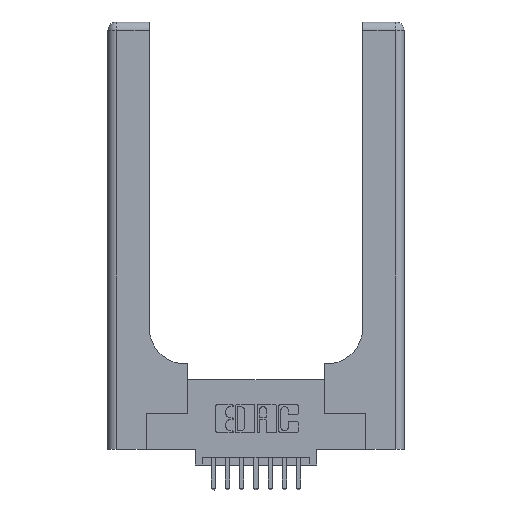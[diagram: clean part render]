
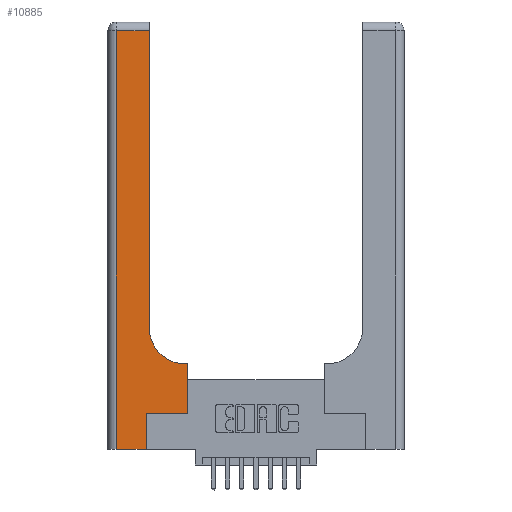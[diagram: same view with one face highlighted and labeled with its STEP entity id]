
A CAD part, top view. The second image highlights one B-rep face of the part: STEP entity #10885.
In plain terms, the highlighted planar face has unit normal (0, 0, 1).
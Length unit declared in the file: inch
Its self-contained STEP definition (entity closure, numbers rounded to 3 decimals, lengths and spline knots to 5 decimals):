
#163 = CARTESIAN_POINT ( 'NONE',  ( 0.2915, 0.85, 0.37 ) ) ;
#548 = VECTOR ( 'NONE', #11658, 39.37008 ) ;
#653 = EDGE_CURVE ( 'NONE', #9798, #8489, #15394, .T. ) ;
#676 = CARTESIAN_POINT ( 'NONE',  ( 0.5415, 0.6, 0.37 ) ) ;
#762 = DIRECTION ( 'NONE',  ( 0., 0., -1. ) ) ;
#998 = EDGE_CURVE ( 'NONE', #1137, #9798, #2732, .T. ) ;
#1020 = CARTESIAN_POINT ( 'NONE',  ( 0., 3., 0.37 ) ) ;
#1137 = VERTEX_POINT ( 'NONE', #5289 ) ;
#2451 = LINE ( 'NONE', #2873, #13931 ) ;
#2629 = CARTESIAN_POINT ( 'NONE',  ( 0., 0., 0.37 ) ) ;
#2639 = VECTOR ( 'NONE', #4273, 39.37008 ) ;
#2732 = LINE ( 'NONE', #12496, #13647 ) ;
#2873 = CARTESIAN_POINT ( 'NONE',  ( 0., 2.94, 0.37 ) ) ;
#3218 = CARTESIAN_POINT ( 'NONE',  ( 0.2915, 3., 0.37 ) ) ;
#3639 = CARTESIAN_POINT ( 'NONE',  ( 0.5585, 0.25, 0.37 ) ) ;
#3951 = CARTESIAN_POINT ( 'NONE',  ( 0.06, 0., 0.37 ) ) ;
#4054 = EDGE_CURVE ( 'NONE', #8489, #8367, #8633, .T. ) ;
#4134 = LINE ( 'NONE', #2629, #6196 ) ;
#4273 = DIRECTION ( 'NONE',  ( 0., -1., 0. ) ) ;
#4312 = CARTESIAN_POINT ( 'NONE',  ( 0.06, 3., 0.37 ) ) ;
#4530 = DIRECTION ( 'NONE',  ( 1., 0., 0. ) ) ;
#4960 = DIRECTION ( 'NONE',  ( -1., 0., 0. ) ) ;
#5221 = ORIENTED_EDGE ( 'NONE', *, *, #13417, .T. ) ;
#5289 = CARTESIAN_POINT ( 'NONE',  ( 0.269, 0.25, 0.37 ) ) ;
#5920 = ORIENTED_EDGE ( 'NONE', *, *, #998, .T. ) ;
#6196 = VECTOR ( 'NONE', #7492, 39.37008 ) ;
#6249 = CARTESIAN_POINT ( 'NONE',  ( 0.06, 2.94, 0.37 ) ) ;
#6356 = EDGE_CURVE ( 'NONE', #7376, #11219, #4134, .T. ) ;
#6432 = CARTESIAN_POINT ( 'NONE',  ( 0.269, 0., 0.37 ) ) ;
#6492 = DIRECTION ( 'NONE',  ( 1., 0., 0. ) ) ;
#6553 = EDGE_CURVE ( 'NONE', #6806, #11095, #15482, .T. ) ;
#6660 = EDGE_CURVE ( 'NONE', #10969, #7376, #9578, .T. ) ;
#6806 = VERTEX_POINT ( 'NONE', #163 ) ;
#6916 = EDGE_CURVE ( 'NONE', #11095, #10969, #2451, .T. ) ;
#6939 = AXIS2_PLACEMENT_3D ( 'NONE', #1020, #9508, #10745 ) ;
#7376 = VERTEX_POINT ( 'NONE', #3951 ) ;
#7492 = DIRECTION ( 'NONE',  ( 1., 0., 0. ) ) ;
#8244 = PLANE ( 'NONE',  #6939 ) ;
#8367 = VERTEX_POINT ( 'NONE', #676 ) ;
#8489 = VERTEX_POINT ( 'NONE', #9107 ) ;
#8633 = LINE ( 'NONE', #9849, #9194 ) ;
#8913 = DIRECTION ( 'NONE',  ( 0., 1., 0. ) ) ;
#8918 = AXIS2_PLACEMENT_3D ( 'NONE', #14039, #762, #4530 ) ;
#9107 = CARTESIAN_POINT ( 'NONE',  ( 0.5585, 0.6, 0.37 ) ) ;
#9115 = DIRECTION ( 'NONE',  ( -1., 0., 0. ) ) ;
#9163 = LINE ( 'NONE', #6432, #11858 ) ;
#9194 = VECTOR ( 'NONE', #4960, 39.37008 ) ;
#9277 = CARTESIAN_POINT ( 'NONE',  ( 0.269, 0., 0.37 ) ) ;
#9410 = ORIENTED_EDGE ( 'NONE', *, *, #6553, .T. ) ;
#9508 = DIRECTION ( 'NONE',  ( 0., 0., -1. ) ) ;
#9578 = LINE ( 'NONE', #4312, #2639 ) ;
#9798 = VERTEX_POINT ( 'NONE', #3639 ) ;
#9849 = CARTESIAN_POINT ( 'NONE',  ( 0.2915, 0.6, 0.37 ) ) ;
#10745 = DIRECTION ( 'NONE',  ( -1., 0., 0. ) ) ;
#10885 = ADVANCED_FACE ( 'NONE', ( #13999 ), #8244, .F. ) ;
#10969 = VERTEX_POINT ( 'NONE', #6249 ) ;
#11095 = VERTEX_POINT ( 'NONE', #11842 ) ;
#11219 = VERTEX_POINT ( 'NONE', #9277 ) ;
#11658 = DIRECTION ( 'NONE',  ( 0., 1., 0. ) ) ;
#11842 = CARTESIAN_POINT ( 'NONE',  ( 0.2915, 2.94, 0.37 ) ) ;
#11858 = VECTOR ( 'NONE', #8913, 39.37008 ) ;
#11937 = EDGE_LOOP ( 'NONE', ( #9410, #11992, #13748, #14980, #5221, #5920, #14969, #13013, #12332 ) ) ;
#11992 = ORIENTED_EDGE ( 'NONE', *, *, #6916, .T. ) ;
#12332 = ORIENTED_EDGE ( 'NONE', *, *, #12562, .T. ) ;
#12496 = CARTESIAN_POINT ( 'NONE',  ( 0.269, 0.25, 0.37 ) ) ;
#12562 = EDGE_CURVE ( 'NONE', #8367, #6806, #14365, .T. ) ;
#13013 = ORIENTED_EDGE ( 'NONE', *, *, #4054, .T. ) ;
#13417 = EDGE_CURVE ( 'NONE', #11219, #1137, #9163, .T. ) ;
#13647 = VECTOR ( 'NONE', #6492, 39.37008 ) ;
#13748 = ORIENTED_EDGE ( 'NONE', *, *, #6660, .T. ) ;
#13931 = VECTOR ( 'NONE', #9115, 39.37008 ) ;
#13999 = FACE_OUTER_BOUND ( 'NONE', #11937, .T. ) ;
#14039 = CARTESIAN_POINT ( 'NONE',  ( 0.5415, 0.85, 0.37 ) ) ;
#14234 = DIRECTION ( 'NONE',  ( 0., 1., 0. ) ) ;
#14285 = CARTESIAN_POINT ( 'NONE',  ( 0.5585, 0.25, 0.37 ) ) ;
#14365 = CIRCLE ( 'NONE', #8918, 0.25 ) ;
#14969 = ORIENTED_EDGE ( 'NONE', *, *, #653, .T. ) ;
#14980 = ORIENTED_EDGE ( 'NONE', *, *, #6356, .T. ) ;
#15003 = VECTOR ( 'NONE', #14234, 39.37008 ) ;
#15394 = LINE ( 'NONE', #14285, #15003 ) ;
#15482 = LINE ( 'NONE', #3218, #548 ) ;
